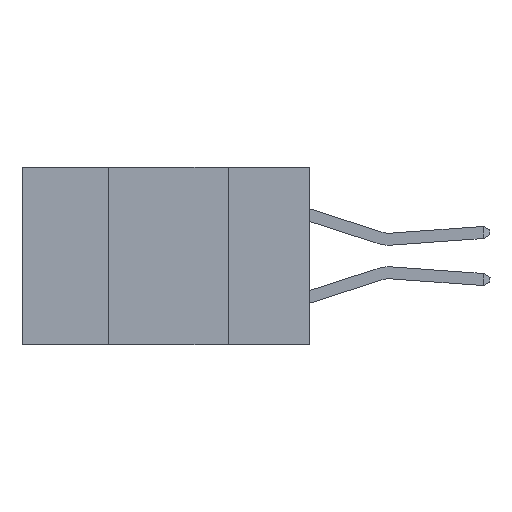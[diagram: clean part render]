
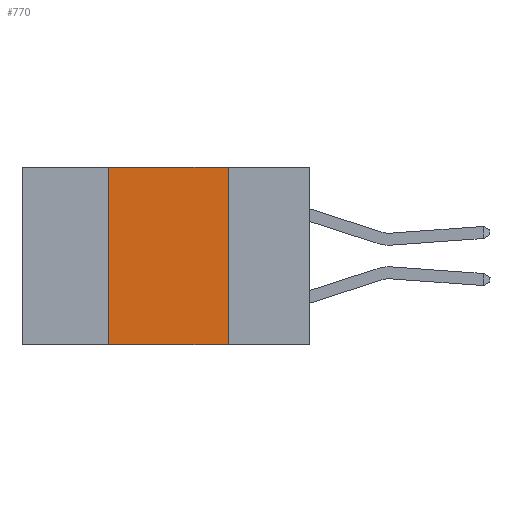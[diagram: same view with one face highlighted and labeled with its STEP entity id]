
A CAD part, left-side view. The second image highlights one B-rep face of the part: STEP entity #770.
In plain terms, the highlighted planar face has unit normal (-1, 0, 0).
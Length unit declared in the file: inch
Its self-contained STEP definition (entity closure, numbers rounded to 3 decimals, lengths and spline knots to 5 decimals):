
#689 = DIRECTION ( 'NONE',  ( 0., -1., 0. ) ) ;
#770 = ADVANCED_FACE ( 'NONE', ( #19353 ), #15312, .F. ) ;
#905 = CARTESIAN_POINT ( 'NONE',  ( 0., 0.6, 0. ) ) ;
#1822 = DIRECTION ( 'NONE',  ( 0., 0., -1. ) ) ;
#2077 = CARTESIAN_POINT ( 'NONE',  ( 0., 0.42, 0. ) ) ;
#2594 = VECTOR ( 'NONE', #689, 39.37008 ) ;
#2988 = EDGE_CURVE ( 'NONE', #13005, #3744, #16395, .T. ) ;
#3204 = LINE ( 'NONE', #14950, #12660 ) ;
#3296 = AXIS2_PLACEMENT_3D ( 'NONE', #17755, #4362, #1822 ) ;
#3729 = ORIENTED_EDGE ( 'NONE', *, *, #6675, .F. ) ;
#3744 = VERTEX_POINT ( 'NONE', #2077 ) ;
#4362 = DIRECTION ( 'NONE',  ( 1., 0., 0. ) ) ;
#4474 = CARTESIAN_POINT ( 'NONE',  ( 0., 0.17, -0.37 ) ) ;
#4935 = VERTEX_POINT ( 'NONE', #21947 ) ;
#5813 = EDGE_CURVE ( 'NONE', #13005, #10294, #3204, .T. ) ;
#6675 = EDGE_CURVE ( 'NONE', #3744, #4935, #21588, .T. ) ;
#10294 = VERTEX_POINT ( 'NONE', #4474 ) ;
#11598 = CARTESIAN_POINT ( 'NONE',  ( 0., 0.42, -0.37 ) ) ;
#12063 = ORIENTED_EDGE ( 'NONE', *, *, #5813, .T. ) ;
#12660 = VECTOR ( 'NONE', #15362, 39.37008 ) ;
#13005 = VERTEX_POINT ( 'NONE', #11598 ) ;
#13257 = LINE ( 'NONE', #22288, #17453 ) ;
#13356 = DIRECTION ( 'NONE',  ( 0., 0., -1. ) ) ;
#13961 = EDGE_LOOP ( 'NONE', ( #17943, #3729, #22149, #12063 ) ) ;
#14950 = CARTESIAN_POINT ( 'NONE',  ( 0., 0.6, -0.37 ) ) ;
#15312 = PLANE ( 'NONE',  #3296 ) ;
#15362 = DIRECTION ( 'NONE',  ( 0., -1., 0. ) ) ;
#16395 = LINE ( 'NONE', #21114, #20633 ) ;
#17453 = VECTOR ( 'NONE', #13356, 39.37008 ) ;
#17755 = CARTESIAN_POINT ( 'NONE',  ( 0., 0.6, 0. ) ) ;
#17943 = ORIENTED_EDGE ( 'NONE', *, *, #22042, .F. ) ;
#19353 = FACE_OUTER_BOUND ( 'NONE', #13961, .T. ) ;
#20633 = VECTOR ( 'NONE', #20699, 39.37008 ) ;
#20699 = DIRECTION ( 'NONE',  ( 0., 0., 1. ) ) ;
#21114 = CARTESIAN_POINT ( 'NONE',  ( 0., 0.42, -0.37 ) ) ;
#21588 = LINE ( 'NONE', #905, #2594 ) ;
#21947 = CARTESIAN_POINT ( 'NONE',  ( 0., 0.17, 0. ) ) ;
#22042 = EDGE_CURVE ( 'NONE', #4935, #10294, #13257, .T. ) ;
#22149 = ORIENTED_EDGE ( 'NONE', *, *, #2988, .F. ) ;
#22288 = CARTESIAN_POINT ( 'NONE',  ( 0., 0.17, -0.37 ) ) ;
